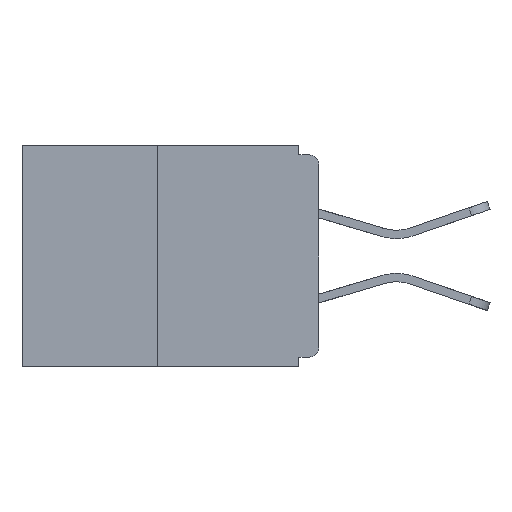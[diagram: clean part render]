
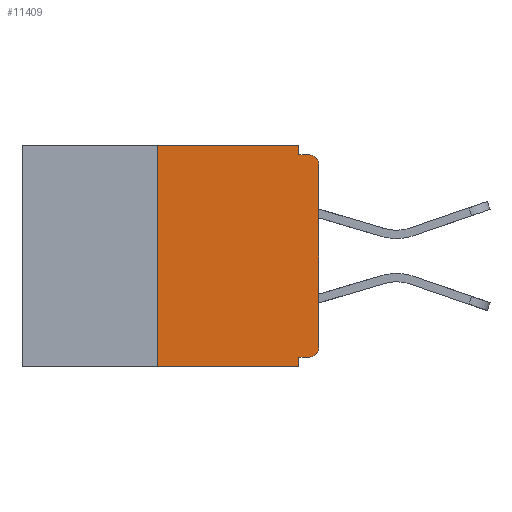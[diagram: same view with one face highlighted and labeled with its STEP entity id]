
A CAD part, left-side view. The second image highlights one B-rep face of the part: STEP entity #11409.
In plain terms, the highlighted planar face has unit normal (-1, 0, 0).
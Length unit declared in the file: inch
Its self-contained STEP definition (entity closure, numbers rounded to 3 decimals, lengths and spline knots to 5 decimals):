
#474 = DIRECTION ( 'NONE',  ( 0., -1., 0. ) ) ;
#1380 = DIRECTION ( 'NONE',  ( -1., 0., 0. ) ) ;
#1409 = FACE_OUTER_BOUND ( 'NONE', #15662, .T. ) ;
#1624 = DIRECTION ( 'NONE',  ( 0., 0., -1. ) ) ;
#1647 = EDGE_CURVE ( 'NONE', #2453, #12390, #10930, .T. ) ;
#1710 = CARTESIAN_POINT ( 'NONE',  ( 0., 0.031, 0. ) ) ;
#1738 = VERTEX_POINT ( 'NONE', #8978 ) ;
#1823 = CARTESIAN_POINT ( 'NONE',  ( 0., 0.46, 0. ) ) ;
#2014 = AXIS2_PLACEMENT_3D ( 'NONE', #5669, #1380, #1624 ) ;
#2160 = EDGE_CURVE ( 'NONE', #8434, #3713, #14246, .T. ) ;
#2453 = VERTEX_POINT ( 'NONE', #13427 ) ;
#2900 = DIRECTION ( 'NONE',  ( 0., 1., 0. ) ) ;
#3418 = DIRECTION ( 'NONE',  ( 0., 0., -1. ) ) ;
#3712 = CARTESIAN_POINT ( 'NONE',  ( 0., 0.015, -0.328 ) ) ;
#3713 = VERTEX_POINT ( 'NONE', #8925 ) ;
#3881 = VERTEX_POINT ( 'NONE', #6869 ) ;
#3939 = DIRECTION ( 'NONE',  ( 0., 0., 1. ) ) ;
#4700 = EDGE_CURVE ( 'NONE', #3881, #14690, #17433, .T. ) ;
#5099 = CARTESIAN_POINT ( 'NONE',  ( 0., 0., -0.015 ) ) ;
#5647 = CARTESIAN_POINT ( 'NONE',  ( 0., 0.031, -0.343 ) ) ;
#5669 = CARTESIAN_POINT ( 'NONE',  ( 0., 0.015, -0.03 ) ) ;
#5869 = DIRECTION ( 'NONE',  ( 0., 0., -1. ) ) ;
#5884 = CARTESIAN_POINT ( 'NONE',  ( 0., 0.031, -0.343 ) ) ;
#6150 = VECTOR ( 'NONE', #14340, 39.37008 ) ;
#6196 = CARTESIAN_POINT ( 'NONE',  ( 0., 0.015, -0.313 ) ) ;
#6634 = DIRECTION ( 'NONE',  ( 0., -1., 0. ) ) ;
#6645 = ORIENTED_EDGE ( 'NONE', *, *, #12674, .F. ) ;
#6716 = CARTESIAN_POINT ( 'NONE',  ( 0., 0., -0.03 ) ) ;
#6869 = CARTESIAN_POINT ( 'NONE',  ( 0., 0.25, -0.343 ) ) ;
#6883 = LINE ( 'NONE', #5099, #8198 ) ;
#7013 = ORIENTED_EDGE ( 'NONE', *, *, #14500, .F. ) ;
#7286 = EDGE_CURVE ( 'NONE', #1738, #8434, #12714, .T. ) ;
#7615 = DIRECTION ( 'NONE',  ( -1., 0., 0. ) ) ;
#8198 = VECTOR ( 'NONE', #6634, 39.37008 ) ;
#8434 = VERTEX_POINT ( 'NONE', #6716 ) ;
#8668 = EDGE_CURVE ( 'NONE', #13010, #1738, #14296, .T. ) ;
#8704 = VECTOR ( 'NONE', #17393, 39.37008 ) ;
#8924 = ORIENTED_EDGE ( 'NONE', *, *, #4700, .T. ) ;
#8925 = CARTESIAN_POINT ( 'NONE',  ( 0., 0.015, -0.015 ) ) ;
#8978 = CARTESIAN_POINT ( 'NONE',  ( 0., 0., -0.313 ) ) ;
#9757 = VECTOR ( 'NONE', #3939, 39.37008 ) ;
#9827 = CARTESIAN_POINT ( 'NONE',  ( 0., 0., -0.328 ) ) ;
#9964 = ORIENTED_EDGE ( 'NONE', *, *, #1647, .F. ) ;
#10003 = LINE ( 'NONE', #5647, #13768 ) ;
#10454 = LINE ( 'NONE', #17341, #8704 ) ;
#10580 = CARTESIAN_POINT ( 'NONE',  ( 0., 0.46, 0. ) ) ;
#10662 = VERTEX_POINT ( 'NONE', #14399 ) ;
#10712 = PLANE ( 'NONE',  #11368 ) ;
#10763 = EDGE_CURVE ( 'NONE', #3881, #2453, #10454, .T. ) ;
#10930 = LINE ( 'NONE', #1823, #6150 ) ;
#11153 = CARTESIAN_POINT ( 'NONE',  ( 0., 0., 0. ) ) ;
#11254 = VECTOR ( 'NONE', #5869, 39.37008 ) ;
#11358 = ORIENTED_EDGE ( 'NONE', *, *, #12735, .F. ) ;
#11368 = AXIS2_PLACEMENT_3D ( 'NONE', #10580, #14886, #16324 ) ;
#11409 = ADVANCED_FACE ( 'NONE', ( #1409 ), #10712, .F. ) ;
#12188 = ORIENTED_EDGE ( 'NONE', *, *, #12317, .F. ) ;
#12317 = EDGE_CURVE ( 'NONE', #14550, #3713, #6883, .T. ) ;
#12390 = VERTEX_POINT ( 'NONE', #17746 ) ;
#12674 = EDGE_CURVE ( 'NONE', #13010, #10662, #15034, .T. ) ;
#12714 = LINE ( 'NONE', #11153, #9757 ) ;
#12735 = EDGE_CURVE ( 'NONE', #12390, #14550, #13060, .T. ) ;
#13010 = VERTEX_POINT ( 'NONE', #3712 ) ;
#13034 = VECTOR ( 'NONE', #2900, 39.37008 ) ;
#13060 = LINE ( 'NONE', #1710, #11254 ) ;
#13427 = CARTESIAN_POINT ( 'NONE',  ( 0., 0.25, 0. ) ) ;
#13768 = VECTOR ( 'NONE', #13983, 39.37008 ) ;
#13916 = VECTOR ( 'NONE', #474, 39.37008 ) ;
#13945 = ORIENTED_EDGE ( 'NONE', *, *, #2160, .T. ) ;
#13983 = DIRECTION ( 'NONE',  ( 0., 0., -1. ) ) ;
#14246 = CIRCLE ( 'NONE', #2014, 0.015 ) ;
#14296 = CIRCLE ( 'NONE', #15788, 0.015 ) ;
#14340 = DIRECTION ( 'NONE',  ( 0., -1., 0. ) ) ;
#14399 = CARTESIAN_POINT ( 'NONE',  ( 0., 0.031, -0.328 ) ) ;
#14500 = EDGE_CURVE ( 'NONE', #10662, #14690, #10003, .T. ) ;
#14550 = VERTEX_POINT ( 'NONE', #18207 ) ;
#14690 = VERTEX_POINT ( 'NONE', #5884 ) ;
#14886 = DIRECTION ( 'NONE',  ( 1., 0., 0. ) ) ;
#15034 = LINE ( 'NONE', #9827, #13034 ) ;
#15662 = EDGE_LOOP ( 'NONE', ( #9964, #15857, #8924, #7013, #6645, #18181, #16568, #13945, #12188, #11358 ) ) ;
#15788 = AXIS2_PLACEMENT_3D ( 'NONE', #6196, #7615, #3418 ) ;
#15857 = ORIENTED_EDGE ( 'NONE', *, *, #10763, .F. ) ;
#16324 = DIRECTION ( 'NONE',  ( 0., 0., -1. ) ) ;
#16568 = ORIENTED_EDGE ( 'NONE', *, *, #7286, .T. ) ;
#17341 = CARTESIAN_POINT ( 'NONE',  ( 0., 0.25, 0. ) ) ;
#17350 = CARTESIAN_POINT ( 'NONE',  ( 0., 0.46, -0.343 ) ) ;
#17393 = DIRECTION ( 'NONE',  ( 0., 0., 1. ) ) ;
#17433 = LINE ( 'NONE', #17350, #13916 ) ;
#17746 = CARTESIAN_POINT ( 'NONE',  ( 0., 0.031, 0. ) ) ;
#18181 = ORIENTED_EDGE ( 'NONE', *, *, #8668, .T. ) ;
#18207 = CARTESIAN_POINT ( 'NONE',  ( 0., 0.031, -0.015 ) ) ;
